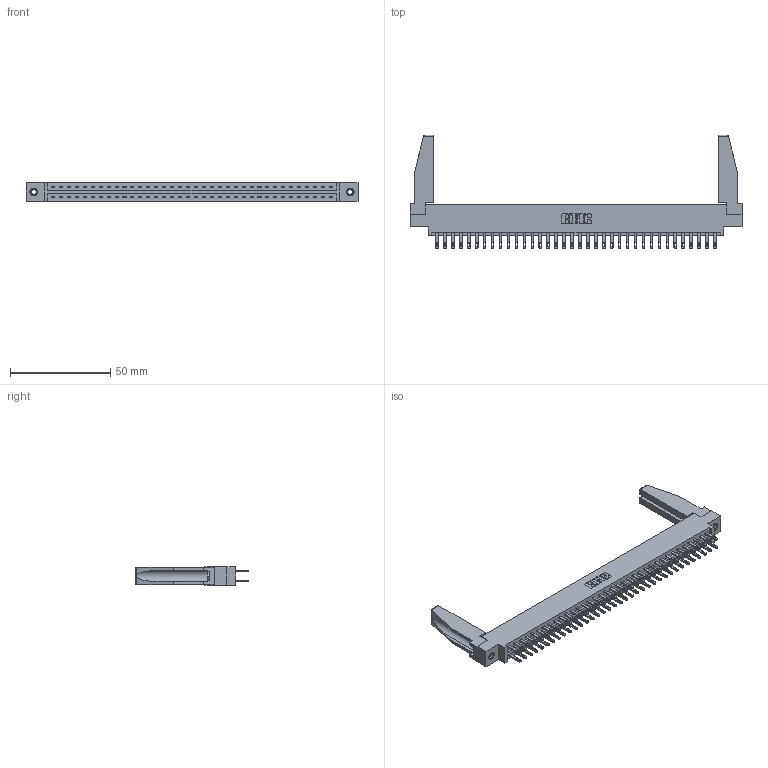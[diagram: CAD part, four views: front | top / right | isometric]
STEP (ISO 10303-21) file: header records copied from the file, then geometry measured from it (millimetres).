
FILE_DESCRIPTION (( 'STEP AP203' ), '1' );
FILE_NAME ('337-072-500-878.STEP', '2019-10-15T11:25:22', ( '' ), ( '' ), 'SwSTEP 2.0', 'SolidWorks 2016', '' );
FILE_SCHEMA (( 'CONFIG_CONTROL_DESIGN' ));
Length unit declared in the file: inch
Products named in the file (5): 337 Part_0.170 Offset - 0.156 Dia-TI; 337-072-500-878; 345-250-001_345-250-001-102; 345-292-001_345-293-100; 307-220-078
Assembly tree (77 placements, depth 2):
  337-072-500-878
    337 Part_0.170 Offset - 0.156 Dia-TI
    345-292-001_345-293-100  x72
    345-250-001_345-250-001-102  x2
    307-220-078  x2
Bounding box: 165.66 x 56.65 x 9.4 mm (x, y, z)
Volume: 21474.4 mm3; surface area: 24441.3 mm2
Topology: 77 solids, 77 shells, 3848 faces, 11669 edges, 7770 vertices
Faces by surface type: plane 2462, cylinder 1370, cone 12, torus 4
Entity records: 31190 total; most frequent: CARTESIAN_POINT 5260, ORIENTED_EDGE 5152, DIRECTION 4492, EDGE_CURVE 2576, VECTOR 2406, LINE 2406, VERTEX_POINT 1712, AXIS2_PLACEMENT_3D 1043
